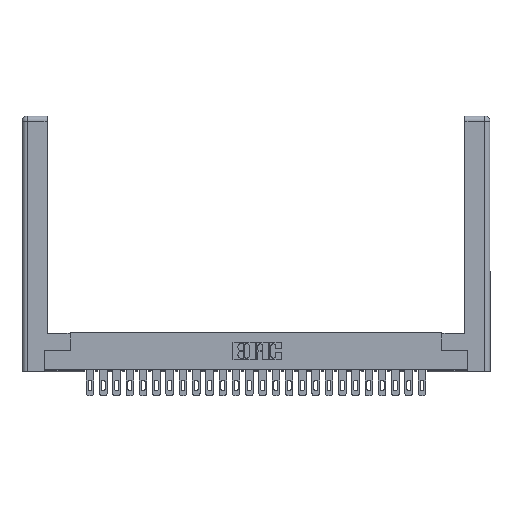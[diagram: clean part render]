
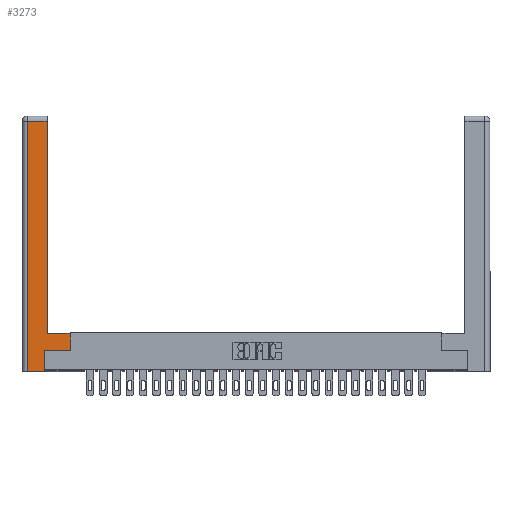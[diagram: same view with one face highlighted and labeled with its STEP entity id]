
A CAD part, top view. The second image highlights one B-rep face of the part: STEP entity #3273.
In plain terms, the highlighted planar face has unit normal (0, 0, 1).
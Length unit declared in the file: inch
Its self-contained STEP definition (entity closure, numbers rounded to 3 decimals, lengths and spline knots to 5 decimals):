
#623 = LINE ( 'NONE', #26311, #9675 ) ;
#1086 = CARTESIAN_POINT ( 'NONE',  ( 0.0615, 2.94, 0. ) ) ;
#1190 = ORIENTED_EDGE ( 'NONE', *, *, #10200, .T. ) ;
#1453 = DIRECTION ( 'NONE',  ( 0., 1., 0. ) ) ;
#1997 = ORIENTED_EDGE ( 'NONE', *, *, #8330, .T. ) ;
#2343 = VECTOR ( 'NONE', #8268, 39.37008 ) ;
#3185 = DIRECTION ( 'NONE',  ( 0., 1., 0. ) ) ;
#3273 = ADVANCED_FACE ( 'NONE', ( #8952 ), #9535, .F. ) ;
#3652 = DIRECTION ( 'NONE',  ( -1., 0., 0. ) ) ;
#3742 = EDGE_CURVE ( 'NONE', #8054, #23169, #24435, .T. ) ;
#4347 = LINE ( 'NONE', #31894, #32425 ) ;
#4734 = CARTESIAN_POINT ( 'NONE',  ( 0., 0., 0. ) ) ;
#4793 = VECTOR ( 'NONE', #1453, 39.37008 ) ;
#5034 = VERTEX_POINT ( 'NONE', #30260 ) ;
#5385 = EDGE_CURVE ( 'NONE', #5034, #27240, #623, .T. ) ;
#6086 = AXIS2_PLACEMENT_3D ( 'NONE', #4734, #29975, #14791 ) ;
#7037 = CARTESIAN_POINT ( 'NONE',  ( 0.295, 2.94, 0. ) ) ;
#7999 = LINE ( 'NONE', #13919, #31796 ) ;
#8054 = VERTEX_POINT ( 'NONE', #22032 ) ;
#8268 = DIRECTION ( 'NONE',  ( 0., -1., 0. ) ) ;
#8330 = EDGE_CURVE ( 'NONE', #27240, #26355, #16615, .T. ) ;
#8390 = CARTESIAN_POINT ( 'NONE',  ( 0.265, 0.245, 0. ) ) ;
#8765 = CARTESIAN_POINT ( 'NONE',  ( 0.565, 0.45, 0. ) ) ;
#8952 = FACE_OUTER_BOUND ( 'NONE', #10127, .T. ) ;
#9061 = VECTOR ( 'NONE', #3652, 39.37008 ) ;
#9535 = PLANE ( 'NONE',  #6086 ) ;
#9675 = VECTOR ( 'NONE', #16203, 39.37008 ) ;
#10127 = EDGE_LOOP ( 'NONE', ( #32776, #1997, #21921, #19231, #25911, #1190, #10358, #13101 ) ) ;
#10200 = EDGE_CURVE ( 'NONE', #23169, #23843, #4347, .T. ) ;
#10358 = ORIENTED_EDGE ( 'NONE', *, *, #30506, .T. ) ;
#10678 = CARTESIAN_POINT ( 'NONE',  ( 0.565, 0.245, 0. ) ) ;
#10873 = EDGE_CURVE ( 'NONE', #26355, #28092, #32389, .T. ) ;
#12178 = CARTESIAN_POINT ( 'NONE',  ( 0.0615, 2.94, 0. ) ) ;
#13101 = ORIENTED_EDGE ( 'NONE', *, *, #16088, .T. ) ;
#13329 = LINE ( 'NONE', #19662, #20852 ) ;
#13567 = CARTESIAN_POINT ( 'NONE',  ( 0.0615, 0., 0. ) ) ;
#13919 = CARTESIAN_POINT ( 'NONE',  ( 0.265, 0., 0. ) ) ;
#13971 = VERTEX_POINT ( 'NONE', #18703 ) ;
#14370 = EDGE_CURVE ( 'NONE', #28092, #8054, #7999, .T. ) ;
#14791 = DIRECTION ( 'NONE',  ( -1., 0., 0. ) ) ;
#16088 = EDGE_CURVE ( 'NONE', #13971, #5034, #13329, .T. ) ;
#16203 = DIRECTION ( 'NONE',  ( 0., 1., 0. ) ) ;
#16615 = LINE ( 'NONE', #1086, #9061 ) ;
#18655 = CARTESIAN_POINT ( 'NONE',  ( 0.265, 0.245, 0. ) ) ;
#18703 = CARTESIAN_POINT ( 'NONE',  ( 0.565, 0.45, 0. ) ) ;
#19231 = ORIENTED_EDGE ( 'NONE', *, *, #14370, .T. ) ;
#19662 = CARTESIAN_POINT ( 'NONE',  ( 0.295, 0.45, 0. ) ) ;
#20852 = VECTOR ( 'NONE', #27228, 39.37008 ) ;
#20895 = VECTOR ( 'NONE', #3185, 39.37008 ) ;
#21921 = ORIENTED_EDGE ( 'NONE', *, *, #10873, .T. ) ;
#22032 = CARTESIAN_POINT ( 'NONE',  ( 0.265, 0., 0. ) ) ;
#23169 = VERTEX_POINT ( 'NONE', #18655 ) ;
#23566 = DIRECTION ( 'NONE',  ( 1., 0., 0. ) ) ;
#23843 = VERTEX_POINT ( 'NONE', #10678 ) ;
#24435 = LINE ( 'NONE', #8390, #20895 ) ;
#25911 = ORIENTED_EDGE ( 'NONE', *, *, #3742, .T. ) ;
#26311 = CARTESIAN_POINT ( 'NONE',  ( 0.295, 3., 0. ) ) ;
#26355 = VERTEX_POINT ( 'NONE', #12178 ) ;
#27228 = DIRECTION ( 'NONE',  ( -1., 0., 0. ) ) ;
#27240 = VERTEX_POINT ( 'NONE', #7037 ) ;
#28092 = VERTEX_POINT ( 'NONE', #13567 ) ;
#28529 = LINE ( 'NONE', #8765, #4793 ) ;
#28656 = DIRECTION ( 'NONE',  ( 1., 0., 0. ) ) ;
#29975 = DIRECTION ( 'NONE',  ( 0., 0., -1. ) ) ;
#30260 = CARTESIAN_POINT ( 'NONE',  ( 0.295, 0.45, 0. ) ) ;
#30506 = EDGE_CURVE ( 'NONE', #23843, #13971, #28529, .T. ) ;
#31015 = CARTESIAN_POINT ( 'NONE',  ( 0.0615, 0., 0. ) ) ;
#31796 = VECTOR ( 'NONE', #28656, 39.37008 ) ;
#31894 = CARTESIAN_POINT ( 'NONE',  ( 0.565, 0.245, 0. ) ) ;
#32389 = LINE ( 'NONE', #31015, #2343 ) ;
#32425 = VECTOR ( 'NONE', #23566, 39.37008 ) ;
#32776 = ORIENTED_EDGE ( 'NONE', *, *, #5385, .T. ) ;
